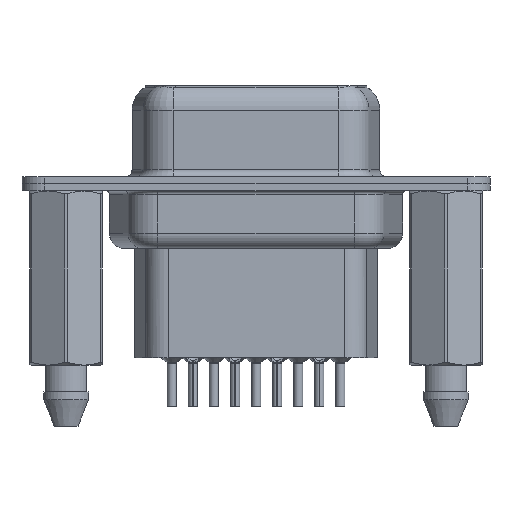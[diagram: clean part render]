
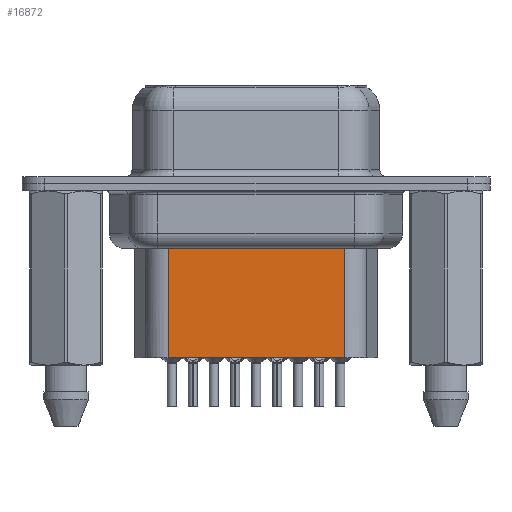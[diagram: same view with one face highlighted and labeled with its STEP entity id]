
A CAD part, front view. The second image highlights one B-rep face of the part: STEP entity #16872.
In plain terms, the highlighted planar face has unit normal (0, -1, 0).
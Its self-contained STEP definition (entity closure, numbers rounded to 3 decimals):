
#45 = ORIENTED_EDGE ( 'NONE', *, *, #5249, .T. ) ;
#83 = EDGE_LOOP ( 'NONE', ( #11168, #45, #4659, #20904 ) ) ;
#953 = VECTOR ( 'NONE', #5918, 1000. ) ;
#2075 = CARTESIAN_POINT ( 'NONE',  ( 6.706, -3.5, -11.45 ) ) ;
#2169 = CARTESIAN_POINT ( 'NONE',  ( 18.294, -3.5, -3.1 ) ) ;
#2443 = VERTEX_POINT ( 'NONE', #5633 ) ;
#2569 = CARTESIAN_POINT ( 'NONE',  ( 6.459, -3.5, -4.097 ) ) ;
#2684 = DIRECTION ( 'NONE',  ( -1., 0., 0. ) ) ;
#3679 = EDGE_CURVE ( 'NONE', #11114, #2443, #10410, .T. ) ;
#4423 = LINE ( 'NONE', #17225, #23724 ) ;
#4626 = CARTESIAN_POINT ( 'NONE',  ( 18.294, -3.5, -4.097 ) ) ;
#4659 = ORIENTED_EDGE ( 'NONE', *, *, #6637, .T. ) ;
#5249 = EDGE_CURVE ( 'NONE', #11114, #8539, #20019, .T. ) ;
#5441 = FACE_OUTER_BOUND ( 'NONE', #83, .T. ) ;
#5633 = CARTESIAN_POINT ( 'NONE',  ( 18.294, -3.5, -11.45 ) ) ;
#5918 = DIRECTION ( 'NONE',  ( 0., 0., -1. ) ) ;
#6637 = EDGE_CURVE ( 'NONE', #8539, #19403, #4423, .T. ) ;
#6874 = DIRECTION ( 'NONE',  ( -1., 0., 0. ) ) ;
#8539 = VERTEX_POINT ( 'NONE', #16772 ) ;
#9220 = DIRECTION ( 'NONE',  ( 0., 0., -1. ) ) ;
#9403 = VECTOR ( 'NONE', #6874, 1000. ) ;
#10410 = LINE ( 'NONE', #2169, #953 ) ;
#10444 = DIRECTION ( 'NONE',  ( 0., -1., 0. ) ) ;
#10599 = EDGE_CURVE ( 'NONE', #2443, #19403, #14418, .T. ) ;
#11114 = VERTEX_POINT ( 'NONE', #4626 ) ;
#11168 = ORIENTED_EDGE ( 'NONE', *, *, #3679, .F. ) ;
#12436 = CARTESIAN_POINT ( 'NONE',  ( 6.706, -3.5, -11.45 ) ) ;
#12778 = PLANE ( 'NONE',  #20763 ) ;
#14418 = LINE ( 'NONE', #12436, #9403 ) ;
#15046 = VECTOR ( 'NONE', #2684, 1000. ) ;
#16530 = CARTESIAN_POINT ( 'NONE',  ( 6.706, -3.5, -3.1 ) ) ;
#16772 = CARTESIAN_POINT ( 'NONE',  ( 6.706, -3.5, -4.097 ) ) ;
#16872 = ADVANCED_FACE ( 'NONE', ( #5441 ), #12778, .T. ) ;
#17225 = CARTESIAN_POINT ( 'NONE',  ( 6.706, -3.5, -3.1 ) ) ;
#19403 = VERTEX_POINT ( 'NONE', #2075 ) ;
#20019 = LINE ( 'NONE', #2569, #15046 ) ;
#20763 = AXIS2_PLACEMENT_3D ( 'NONE', #16530, #10444, #23506 ) ;
#20904 = ORIENTED_EDGE ( 'NONE', *, *, #10599, .F. ) ;
#23506 = DIRECTION ( 'NONE',  ( 1., 0., 0. ) ) ;
#23724 = VECTOR ( 'NONE', #9220, 1000. ) ;
